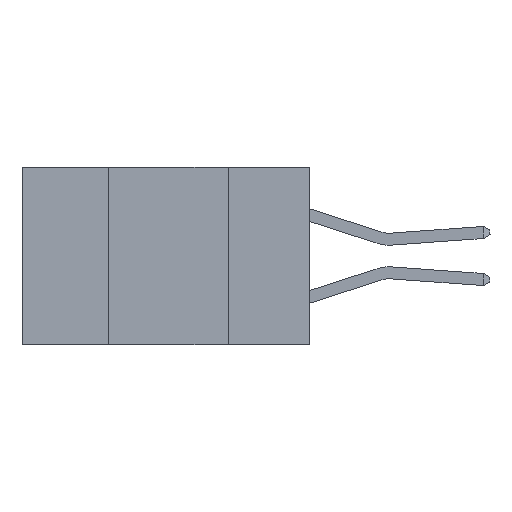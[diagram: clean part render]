
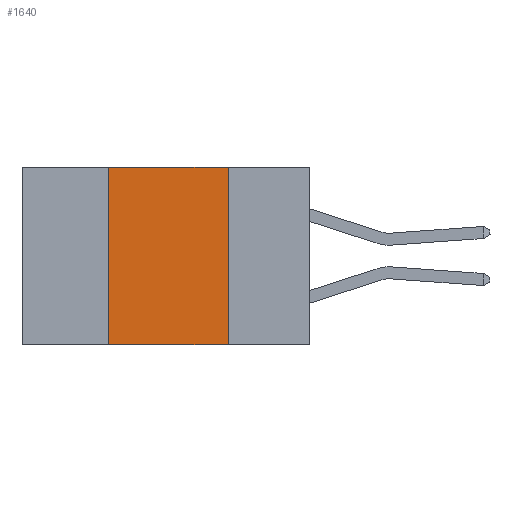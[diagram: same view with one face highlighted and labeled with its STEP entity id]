
A CAD part, left-side view. The second image highlights one B-rep face of the part: STEP entity #1640.
In plain terms, the highlighted planar face has unit normal (-1, 0, 0).
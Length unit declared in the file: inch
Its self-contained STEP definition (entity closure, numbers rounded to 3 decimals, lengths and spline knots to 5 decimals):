
#655 = CARTESIAN_POINT ( 'NONE',  ( 0., 0.6, 0. ) ) ;
#948 = AXIS2_PLACEMENT_3D ( 'NONE', #655, #4126, #2995 ) ;
#1640 = ADVANCED_FACE ( 'NONE', ( #14412 ), #14551, .F. ) ;
#2443 = DIRECTION ( 'NONE',  ( 0., 0., -1. ) ) ;
#2482 = VECTOR ( 'NONE', #12618, 39.37008 ) ;
#2668 = LINE ( 'NONE', #10436, #7835 ) ;
#2711 = CARTESIAN_POINT ( 'NONE',  ( 0., 0.17, -0.37 ) ) ;
#2995 = DIRECTION ( 'NONE',  ( 0., 0., -1. ) ) ;
#3378 = LINE ( 'NONE', #3673, #4849 ) ;
#3403 = LINE ( 'NONE', #6818, #2482 ) ;
#3673 = CARTESIAN_POINT ( 'NONE',  ( 0., 0.6, 0. ) ) ;
#4126 = DIRECTION ( 'NONE',  ( 1., 0., 0. ) ) ;
#4849 = VECTOR ( 'NONE', #14172, 39.37008 ) ;
#5223 = VERTEX_POINT ( 'NONE', #5625 ) ;
#5625 = CARTESIAN_POINT ( 'NONE',  ( 0., 0.42, -0.37 ) ) ;
#5670 = ORIENTED_EDGE ( 'NONE', *, *, #13419, .F. ) ;
#6098 = ORIENTED_EDGE ( 'NONE', *, *, #11040, .F. ) ;
#6490 = CARTESIAN_POINT ( 'NONE',  ( 0., 0.17, 0. ) ) ;
#6818 = CARTESIAN_POINT ( 'NONE',  ( 0., 0.6, -0.37 ) ) ;
#6953 = ORIENTED_EDGE ( 'NONE', *, *, #12093, .T. ) ;
#7357 = LINE ( 'NONE', #10685, #9071 ) ;
#7426 = VERTEX_POINT ( 'NONE', #13110 ) ;
#7835 = VECTOR ( 'NONE', #2443, 39.37008 ) ;
#9071 = VECTOR ( 'NONE', #13023, 39.37008 ) ;
#9603 = EDGE_LOOP ( 'NONE', ( #5670, #6098, #14574, #6953 ) ) ;
#9793 = VERTEX_POINT ( 'NONE', #2711 ) ;
#10436 = CARTESIAN_POINT ( 'NONE',  ( 0., 0.17, -0.37 ) ) ;
#10685 = CARTESIAN_POINT ( 'NONE',  ( 0., 0.42, -0.37 ) ) ;
#11040 = EDGE_CURVE ( 'NONE', #7426, #12968, #3378, .T. ) ;
#12093 = EDGE_CURVE ( 'NONE', #5223, #9793, #3403, .T. ) ;
#12618 = DIRECTION ( 'NONE',  ( 0., -1., 0. ) ) ;
#12968 = VERTEX_POINT ( 'NONE', #6490 ) ;
#13023 = DIRECTION ( 'NONE',  ( 0., 0., 1. ) ) ;
#13110 = CARTESIAN_POINT ( 'NONE',  ( 0., 0.42, 0. ) ) ;
#13419 = EDGE_CURVE ( 'NONE', #12968, #9793, #2668, .T. ) ;
#14172 = DIRECTION ( 'NONE',  ( 0., -1., 0. ) ) ;
#14412 = FACE_OUTER_BOUND ( 'NONE', #9603, .T. ) ;
#14551 = PLANE ( 'NONE',  #948 ) ;
#14560 = EDGE_CURVE ( 'NONE', #5223, #7426, #7357, .T. ) ;
#14574 = ORIENTED_EDGE ( 'NONE', *, *, #14560, .F. ) ;
